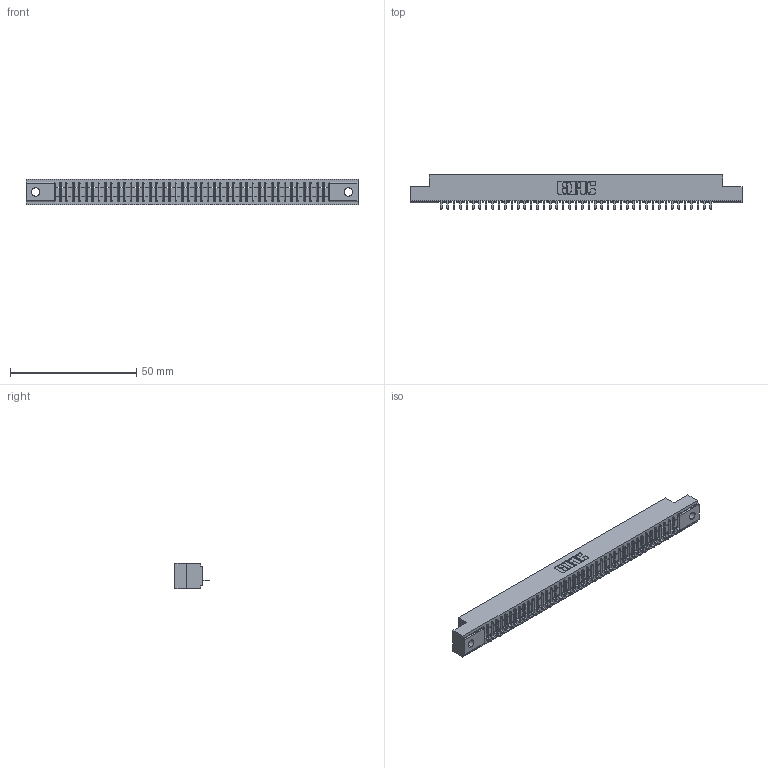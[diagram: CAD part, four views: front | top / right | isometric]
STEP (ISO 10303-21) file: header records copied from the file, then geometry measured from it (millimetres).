
FILE_DESCRIPTION (( 'STEP AP203' ), '1' );
FILE_NAME ('391-043-524-102.STEP', '2018-08-09T02:10:03', ( '' ), ( '' ), 'SwSTEP 2.0', 'SolidWorks 2016', '' );
FILE_SCHEMA (( 'CONFIG_CONTROL_DESIGN' ));
Length unit declared in the file: inch
Products named in the file (3): 341 Part_.128 (3.25) Dia Mounting Holes; 341-292-001_341-292-124; 391-043-524-102
Assembly tree (44 placements, depth 2):
  391-043-524-102
    341 Part_.128 (3.25) Dia Mounting Holes
    341-292-001_341-292-124  x43
Bounding box: 131.44 x 13.64 x 10.16 mm (x, y, z)
Volume: 9355.5 mm3; surface area: 14163.9 mm2
Topology: 44 solids, 44 shells, 3642 faces, 10507 edges, 6742 vertices
Faces by surface type: plane 2261, cylinder 1209, sphere 88, torus 84
Entity records: 50532 total; most frequent: CARTESIAN_POINT 8586, ORIENTED_EDGE 8574, DIRECTION 8287, EDGE_CURVE 4287, LINE 3465, VECTOR 3465, VERTEX_POINT 2710, AXIS2_PLACEMENT_3D 2411
